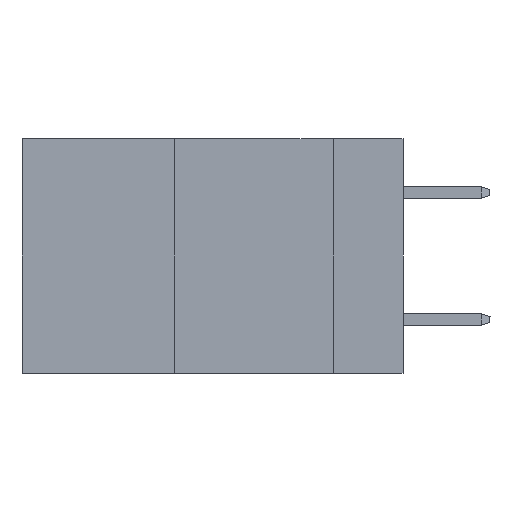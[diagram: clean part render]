
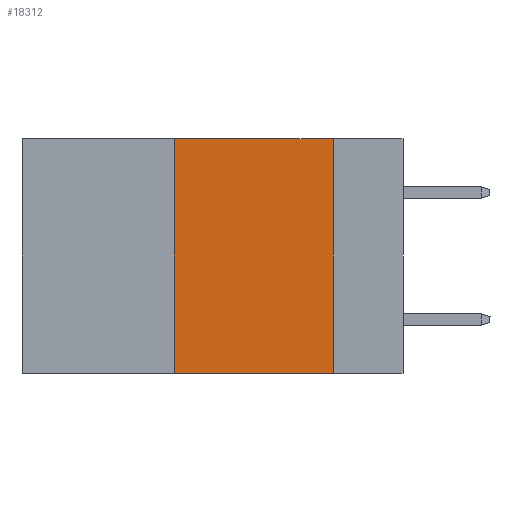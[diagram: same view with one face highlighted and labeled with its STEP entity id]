
A CAD part, left-side view. The second image highlights one B-rep face of the part: STEP entity #18312.
In plain terms, the highlighted planar face has unit normal (-1, 0, 0).
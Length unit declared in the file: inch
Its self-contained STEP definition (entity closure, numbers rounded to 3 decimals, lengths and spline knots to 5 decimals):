
#1406 = LINE ( 'NONE', #26343, #19568 ) ;
#1464 = DIRECTION ( 'NONE',  ( 0., 0., -1. ) ) ;
#2515 = VECTOR ( 'NONE', #8773, 39.37008 ) ;
#3006 = ORIENTED_EDGE ( 'NONE', *, *, #24196, .F. ) ;
#3646 = EDGE_CURVE ( 'NONE', #7050, #13827, #5637, .T. ) ;
#4502 = LINE ( 'NONE', #20644, #2515 ) ;
#4869 = VERTEX_POINT ( 'NONE', #5572 ) ;
#5572 = CARTESIAN_POINT ( 'NONE',  ( 0., 0.36, 0. ) ) ;
#5637 = LINE ( 'NONE', #19109, #21978 ) ;
#5653 = CARTESIAN_POINT ( 'NONE',  ( 0., 0.11, -0.37 ) ) ;
#6296 = CARTESIAN_POINT ( 'NONE',  ( 0., 0.11, 0. ) ) ;
#6317 = DIRECTION ( 'NONE',  ( 1., 0., 0. ) ) ;
#6458 = FACE_OUTER_BOUND ( 'NONE', #7343, .T. ) ;
#7050 = VERTEX_POINT ( 'NONE', #19118 ) ;
#7343 = EDGE_LOOP ( 'NONE', ( #3006, #8041, #27678, #14835 ) ) ;
#7973 = DIRECTION ( 'NONE',  ( 0., -1., 0. ) ) ;
#8041 = ORIENTED_EDGE ( 'NONE', *, *, #22981, .F. ) ;
#8392 = CARTESIAN_POINT ( 'NONE',  ( 0., 0.11, 0. ) ) ;
#8773 = DIRECTION ( 'NONE',  ( 0., -1., 0. ) ) ;
#11053 = PLANE ( 'NONE',  #28425 ) ;
#13128 = CARTESIAN_POINT ( 'NONE',  ( 0., 0.6, 0. ) ) ;
#13827 = VERTEX_POINT ( 'NONE', #5653 ) ;
#14738 = VERTEX_POINT ( 'NONE', #8392 ) ;
#14835 = ORIENTED_EDGE ( 'NONE', *, *, #3646, .T. ) ;
#17878 = DIRECTION ( 'NONE',  ( 0., 0., -1. ) ) ;
#18312 = ADVANCED_FACE ( 'NONE', ( #6458 ), #11053, .F. ) ;
#19109 = CARTESIAN_POINT ( 'NONE',  ( 0., 0.6, -0.37 ) ) ;
#19118 = CARTESIAN_POINT ( 'NONE',  ( 0., 0.36, -0.37 ) ) ;
#19568 = VECTOR ( 'NONE', #21494, 39.37008 ) ;
#20644 = CARTESIAN_POINT ( 'NONE',  ( 0., 0.6, 0. ) ) ;
#20726 = EDGE_CURVE ( 'NONE', #7050, #4869, #1406, .T. ) ;
#21494 = DIRECTION ( 'NONE',  ( 0., 0., 1. ) ) ;
#21978 = VECTOR ( 'NONE', #7973, 39.37008 ) ;
#22981 = EDGE_CURVE ( 'NONE', #4869, #14738, #4502, .T. ) ;
#23346 = VECTOR ( 'NONE', #1464, 39.37008 ) ;
#24196 = EDGE_CURVE ( 'NONE', #14738, #13827, #26553, .T. ) ;
#26343 = CARTESIAN_POINT ( 'NONE',  ( 0., 0.36, 0. ) ) ;
#26553 = LINE ( 'NONE', #6296, #23346 ) ;
#27678 = ORIENTED_EDGE ( 'NONE', *, *, #20726, .F. ) ;
#28425 = AXIS2_PLACEMENT_3D ( 'NONE', #13128, #6317, #17878 ) ;
